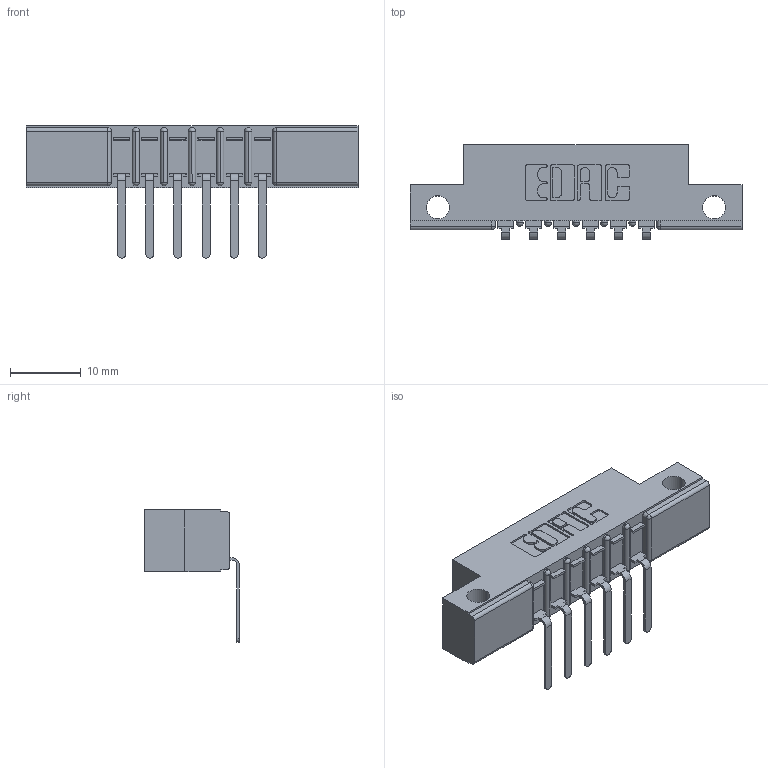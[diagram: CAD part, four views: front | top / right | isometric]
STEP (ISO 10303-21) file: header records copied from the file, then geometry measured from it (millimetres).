
FILE_DESCRIPTION (( 'STEP AP203' ), '1' );
FILE_NAME ('357-006-457-112.STEP', '2020-09-30T01:06:32', ( '' ), ( '' ), 'SwSTEP 2.0', 'SolidWorks 2020', '' );
FILE_SCHEMA (( 'CONFIG_CONTROL_DESIGN' ));
Length unit declared in the file: inch
Products named in the file (3): 357-006-457-112; 307 Part_.128 Dia Side Mounting Holes; 307-290-002_557
Assembly tree (7 placements, depth 2):
  357-006-457-112
    307 Part_.128 Dia Side Mounting Holes
    307-290-002_557  x6
Bounding box: 46.79 x 13.32 x 18.67 mm (x, y, z)
Volume: 3020.7 mm3; surface area: 4565.8 mm2
Topology: 7 solids, 7 shells, 593 faces, 1787 edges, 1170 vertices
Faces by surface type: plane 352, cylinder 227, sphere 14
Entity records: 10438 total; most frequent: CARTESIAN_POINT 1756, ORIENTED_EDGE 1746, DIRECTION 1723, EDGE_CURVE 873, VECTOR 649, LINE 649, VERTEX_POINT 570, AXIS2_PLACEMENT_3D 537
